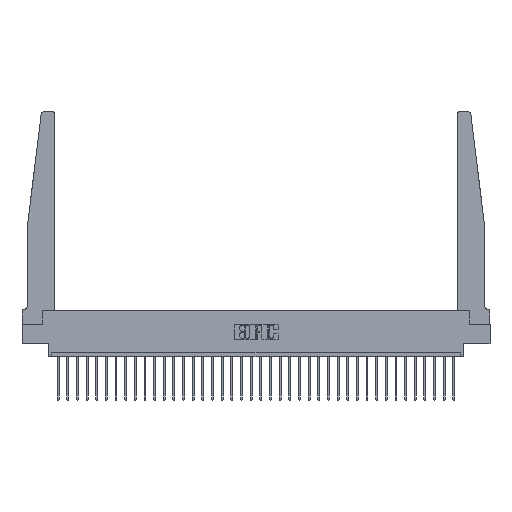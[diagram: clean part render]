
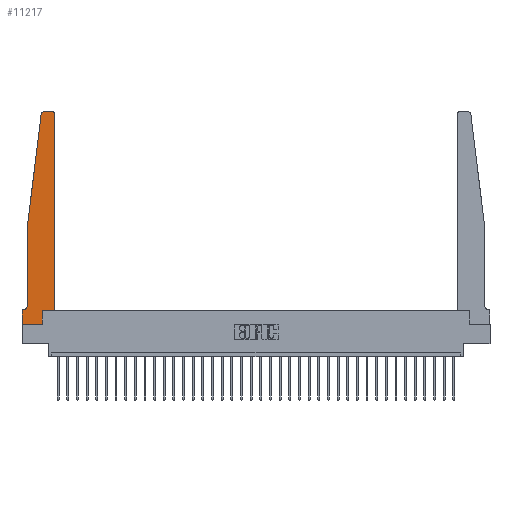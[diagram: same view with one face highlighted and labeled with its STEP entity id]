
A CAD part, top view. The second image highlights one B-rep face of the part: STEP entity #11217.
In plain terms, the highlighted planar face has unit normal (0, 0, 1).
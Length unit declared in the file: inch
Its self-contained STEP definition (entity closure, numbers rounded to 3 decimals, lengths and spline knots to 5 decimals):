
#461 = CARTESIAN_POINT ( 'NONE',  ( 0.425, 0.18, 0.37 ) ) ;
#780 = CARTESIAN_POINT ( 'NONE',  ( 0., 0., 0.37 ) ) ;
#1082 = VERTEX_POINT ( 'NONE', #11948 ) ;
#1909 = CIRCLE ( 'NONE', #9152, 0.03 ) ;
#2675 = DIRECTION ( 'NONE',  ( 1., 0., 0. ) ) ;
#2736 = ORIENTED_EDGE ( 'NONE', *, *, #5710, .T. ) ;
#2771 = DIRECTION ( 'NONE',  ( 0., 0., 1. ) ) ;
#3077 = CARTESIAN_POINT ( 'NONE',  ( 0.24675, 2.72367, 0.37 ) ) ;
#3171 = EDGE_LOOP ( 'NONE', ( #22742, #2736, #6399, #23108, #12311, #11398, #30732, #21625, #3965, #12372, #22072, #12031 ) ) ;
#3237 = DIRECTION ( 'NONE',  ( -1., 0., 0. ) ) ;
#3278 = DIRECTION ( 'NONE',  ( 1., 0., 0. ) ) ;
#3421 = DIRECTION ( 'NONE',  ( -1., 0., 0. ) ) ;
#3429 = CARTESIAN_POINT ( 'NONE',  ( 0., 0.1875, 0.37 ) ) ;
#3472 = EDGE_CURVE ( 'NONE', #7969, #10792, #24231, .T. ) ;
#3890 = EDGE_CURVE ( 'NONE', #12852, #7969, #9945, .T. ) ;
#3965 = ORIENTED_EDGE ( 'NONE', *, *, #3890, .T. ) ;
#4878 = VECTOR ( 'NONE', #9872, 39.37008 ) ;
#5710 = EDGE_CURVE ( 'NONE', #9900, #24941, #21445, .T. ) ;
#5981 = LINE ( 'NONE', #23944, #4878 ) ;
#6199 = EDGE_CURVE ( 'NONE', #13793, #26673, #9409, .T. ) ;
#6399 = ORIENTED_EDGE ( 'NONE', *, *, #28562, .T. ) ;
#7037 = VECTOR ( 'NONE', #3421, 39.37008 ) ;
#7937 = AXIS2_PLACEMENT_3D ( 'NONE', #10288, #17589, #3237 ) ;
#7969 = VERTEX_POINT ( 'NONE', #18381 ) ;
#8720 = EDGE_CURVE ( 'NONE', #10792, #9709, #5981, .T. ) ;
#8968 = DIRECTION ( 'NONE',  ( 0., 1., 0. ) ) ;
#8988 = LINE ( 'NONE', #780, #9736 ) ;
#9152 = AXIS2_PLACEMENT_3D ( 'NONE', #12335, #2771, #24280 ) ;
#9399 = DIRECTION ( 'NONE',  ( 0., 0., 1. ) ) ;
#9409 = LINE ( 'NONE', #30262, #30050 ) ;
#9709 = VERTEX_POINT ( 'NONE', #16342 ) ;
#9736 = VECTOR ( 'NONE', #3278, 39.37008 ) ;
#9872 = DIRECTION ( 'NONE',  ( 0., 1., 0. ) ) ;
#9900 = VERTEX_POINT ( 'NONE', #14938 ) ;
#9945 = LINE ( 'NONE', #13797, #24205 ) ;
#10288 = CARTESIAN_POINT ( 'NONE',  ( 0.015, 0.2375, 0.37 ) ) ;
#10792 = VERTEX_POINT ( 'NONE', #24169 ) ;
#11086 = EDGE_CURVE ( 'NONE', #26673, #24290, #11718, .T. ) ;
#11114 = DIRECTION ( 'NONE',  ( -1., 0., 0. ) ) ;
#11154 = AXIS2_PLACEMENT_3D ( 'NONE', #29309, #19691, #14984 ) ;
#11217 = ADVANCED_FACE ( 'NONE', ( #26701 ), #12523, .T. ) ;
#11294 = VERTEX_POINT ( 'NONE', #12203 ) ;
#11398 = ORIENTED_EDGE ( 'NONE', *, *, #24573, .T. ) ;
#11718 = CIRCLE ( 'NONE', #7937, 0.05 ) ;
#11807 = DIRECTION ( 'NONE',  ( 1., 0., 0. ) ) ;
#11948 = CARTESIAN_POINT ( 'NONE',  ( 0.395, 2.75, 0.37 ) ) ;
#12031 = ORIENTED_EDGE ( 'NONE', *, *, #24798, .T. ) ;
#12137 = DIRECTION ( 'NONE',  ( 0., -1., 0. ) ) ;
#12203 = CARTESIAN_POINT ( 'NONE',  ( 0., 0., 0.37 ) ) ;
#12311 = ORIENTED_EDGE ( 'NONE', *, *, #11086, .T. ) ;
#12335 = CARTESIAN_POINT ( 'NONE',  ( 0.395, 2.72, 0.37 ) ) ;
#12372 = ORIENTED_EDGE ( 'NONE', *, *, #3472, .T. ) ;
#12523 = PLANE ( 'NONE',  #11154 ) ;
#12768 = EDGE_CURVE ( 'NONE', #11294, #12852, #8988, .T. ) ;
#12852 = VERTEX_POINT ( 'NONE', #23077 ) ;
#13680 = VECTOR ( 'NONE', #15517, 39.37008 ) ;
#13793 = VERTEX_POINT ( 'NONE', #15274 ) ;
#13797 = CARTESIAN_POINT ( 'NONE',  ( 0.2605, 0.18, 0.37 ) ) ;
#14191 = LINE ( 'NONE', #21686, #18766 ) ;
#14938 = CARTESIAN_POINT ( 'NONE',  ( 0.27653, 2.75, 0.37 ) ) ;
#14984 = DIRECTION ( 'NONE',  ( 1., 0., 0. ) ) ;
#15274 = CARTESIAN_POINT ( 'NONE',  ( 0.065, 1.25, 0.37 ) ) ;
#15346 = CARTESIAN_POINT ( 'NONE',  ( 0.25, 2.75, 0.37 ) ) ;
#15517 = DIRECTION ( 'NONE',  ( -0.122, -0.992, 0. ) ) ;
#15854 = EDGE_CURVE ( 'NONE', #1082, #9900, #19783, .T. ) ;
#16037 = CARTESIAN_POINT ( 'NONE',  ( 0.065, 0.2375, 0.37 ) ) ;
#16342 = CARTESIAN_POINT ( 'NONE',  ( 0.425, 2.72, 0.37 ) ) ;
#16539 = VECTOR ( 'NONE', #11114, 39.37008 ) ;
#16598 = CARTESIAN_POINT ( 'NONE',  ( 0.27653, 2.72, 0.37 ) ) ;
#17589 = DIRECTION ( 'NONE',  ( 0., 0., -1. ) ) ;
#17730 = CARTESIAN_POINT ( 'NONE',  ( 0.065, 1.25, 0.37 ) ) ;
#18284 = VECTOR ( 'NONE', #2675, 39.37008 ) ;
#18381 = CARTESIAN_POINT ( 'NONE',  ( 0.2605, 0.18, 0.37 ) ) ;
#18766 = VECTOR ( 'NONE', #12137, 39.37008 ) ;
#19603 = VERTEX_POINT ( 'NONE', #3429 ) ;
#19691 = DIRECTION ( 'NONE',  ( 0., 0., 1. ) ) ;
#19783 = LINE ( 'NONE', #15346, #7037 ) ;
#20439 = EDGE_CURVE ( 'NONE', #19603, #11294, #14191, .T. ) ;
#20533 = DIRECTION ( 'NONE',  ( 0., -1., 0. ) ) ;
#21445 = CIRCLE ( 'NONE', #26334, 0.03 ) ;
#21625 = ORIENTED_EDGE ( 'NONE', *, *, #12768, .T. ) ;
#21686 = CARTESIAN_POINT ( 'NONE',  ( 0., 0., 0.37 ) ) ;
#22072 = ORIENTED_EDGE ( 'NONE', *, *, #8720, .T. ) ;
#22742 = ORIENTED_EDGE ( 'NONE', *, *, #15854, .T. ) ;
#22847 = LINE ( 'NONE', #25667, #16539 ) ;
#23077 = CARTESIAN_POINT ( 'NONE',  ( 0.2605, 0., 0.37 ) ) ;
#23108 = ORIENTED_EDGE ( 'NONE', *, *, #6199, .T. ) ;
#23944 = CARTESIAN_POINT ( 'NONE',  ( 0.425, 0.18, 0.37 ) ) ;
#24169 = CARTESIAN_POINT ( 'NONE',  ( 0.425, 0.18, 0.37 ) ) ;
#24205 = VECTOR ( 'NONE', #8968, 39.37008 ) ;
#24231 = LINE ( 'NONE', #461, #18284 ) ;
#24280 = DIRECTION ( 'NONE',  ( 1., 0., 0. ) ) ;
#24290 = VERTEX_POINT ( 'NONE', #24637 ) ;
#24573 = EDGE_CURVE ( 'NONE', #24290, #19603, #22847, .T. ) ;
#24637 = CARTESIAN_POINT ( 'NONE',  ( 0.015, 0.1875, 0.37 ) ) ;
#24798 = EDGE_CURVE ( 'NONE', #9709, #1082, #1909, .T. ) ;
#24941 = VERTEX_POINT ( 'NONE', #3077 ) ;
#25667 = CARTESIAN_POINT ( 'NONE',  ( 0.065, 0.1875, 0.37 ) ) ;
#26334 = AXIS2_PLACEMENT_3D ( 'NONE', #16598, #9399, #11807 ) ;
#26673 = VERTEX_POINT ( 'NONE', #16037 ) ;
#26701 = FACE_OUTER_BOUND ( 'NONE', #3171, .T. ) ;
#28562 = EDGE_CURVE ( 'NONE', #24941, #13793, #29789, .T. ) ;
#29309 = CARTESIAN_POINT ( 'NONE',  ( 0., 0.1875, 0.37 ) ) ;
#29789 = LINE ( 'NONE', #17730, #13680 ) ;
#30050 = VECTOR ( 'NONE', #20533, 39.37008 ) ;
#30262 = CARTESIAN_POINT ( 'NONE',  ( 0.065, 1.25, 0.37 ) ) ;
#30732 = ORIENTED_EDGE ( 'NONE', *, *, #20439, .T. ) ;
